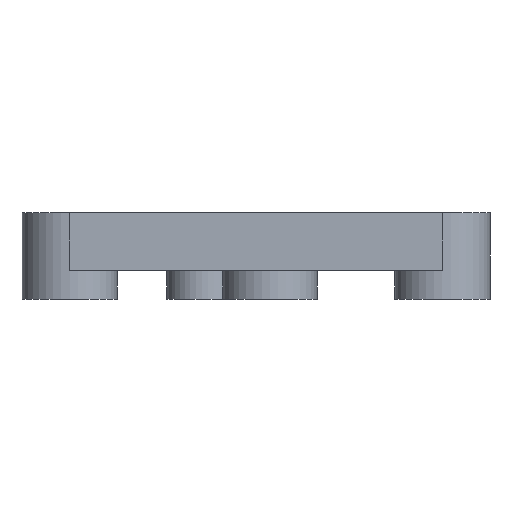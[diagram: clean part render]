
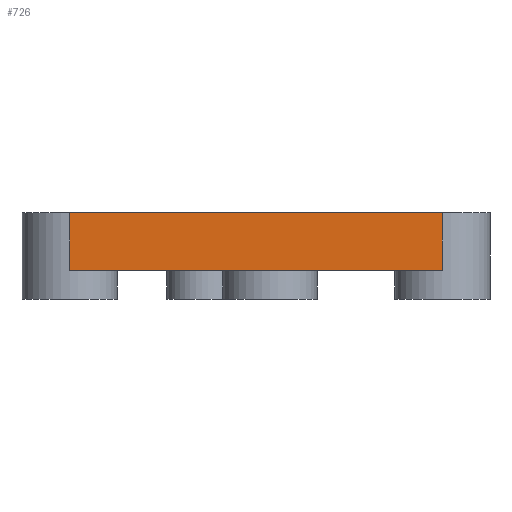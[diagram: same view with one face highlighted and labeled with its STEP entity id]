
A CAD part, front view. The second image highlights one B-rep face of the part: STEP entity #726.
In plain terms, the highlighted planar face has unit normal (0, -1, 0).
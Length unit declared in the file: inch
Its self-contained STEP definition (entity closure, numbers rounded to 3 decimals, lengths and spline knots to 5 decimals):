
#1 = EDGE_CURVE ( 'NONE', #870, #305, #763, .T. ) ;
#20 = EDGE_CURVE ( 'NONE', #666, #870, #854, .T. ) ;
#31 = EDGE_CURVE ( 'NONE', #666, #1094, #1091, .T. ) ;
#38 = DIRECTION ( 'NONE',  ( -1., 0., 0. ) ) ;
#46 = DIRECTION ( 'NONE',  ( 0., 1., 0. ) ) ;
#129 = CARTESIAN_POINT ( 'NONE',  ( 40.119, 4.32089, -2. ) ) ;
#135 = ORIENTED_EDGE ( 'NONE', *, *, #1, .F. ) ;
#137 = PLANE ( 'NONE',  #598 ) ;
#212 = ORIENTED_EDGE ( 'NONE', *, *, #20, .F. ) ;
#227 = DIRECTION ( 'NONE',  ( 0., 0., 1. ) ) ;
#305 = VERTEX_POINT ( 'NONE', #597 ) ;
#329 = CARTESIAN_POINT ( 'NONE',  ( 0., 4.32089, -2. ) ) ;
#345 = ORIENTED_EDGE ( 'NONE', *, *, #31, .T. ) ;
#390 = EDGE_LOOP ( 'NONE', ( #437, #135, #212, #345 ) ) ;
#421 = VECTOR ( 'NONE', #914, 39.37008 ) ;
#436 = CARTESIAN_POINT ( 'NONE',  ( 27.24165, 4.32089, -2. ) ) ;
#437 = ORIENTED_EDGE ( 'NONE', *, *, #756, .T. ) ;
#439 = DIRECTION ( 'NONE',  ( -1., 0., 0. ) ) ;
#478 = CARTESIAN_POINT ( 'NONE',  ( 0., 4.32089, -2. ) ) ;
#495 = VECTOR ( 'NONE', #539, 39.37008 ) ;
#539 = DIRECTION ( 'NONE',  ( 0., 0., 1. ) ) ;
#557 = LINE ( 'NONE', #926, #421 ) ;
#584 = VECTOR ( 'NONE', #439, 39.37008 ) ;
#597 = CARTESIAN_POINT ( 'NONE',  ( 27.24165, 4.32089, 0. ) ) ;
#598 = AXIS2_PLACEMENT_3D ( 'NONE', #478, #46, #38 ) ;
#615 = CARTESIAN_POINT ( 'NONE',  ( 27.24165, 4.32089, -2. ) ) ;
#666 = VERTEX_POINT ( 'NONE', #681 ) ;
#681 = CARTESIAN_POINT ( 'NONE',  ( 40.119, 4.32089, -2. ) ) ;
#684 = CARTESIAN_POINT ( 'NONE',  ( 40.119, 4.32089, 0. ) ) ;
#726 = ADVANCED_FACE ( 'NONE', ( #1103 ), #137, .F. ) ;
#756 = EDGE_CURVE ( 'NONE', #1094, #305, #557, .T. ) ;
#763 = LINE ( 'NONE', #436, #495 ) ;
#822 = VECTOR ( 'NONE', #227, 39.37008 ) ;
#854 = LINE ( 'NONE', #329, #584 ) ;
#870 = VERTEX_POINT ( 'NONE', #615 ) ;
#914 = DIRECTION ( 'NONE',  ( -1., 0., 0. ) ) ;
#926 = CARTESIAN_POINT ( 'NONE',  ( 0., 4.32089, 0. ) ) ;
#1091 = LINE ( 'NONE', #129, #822 ) ;
#1094 = VERTEX_POINT ( 'NONE', #684 ) ;
#1103 = FACE_OUTER_BOUND ( 'NONE', #390, .T. ) ;
